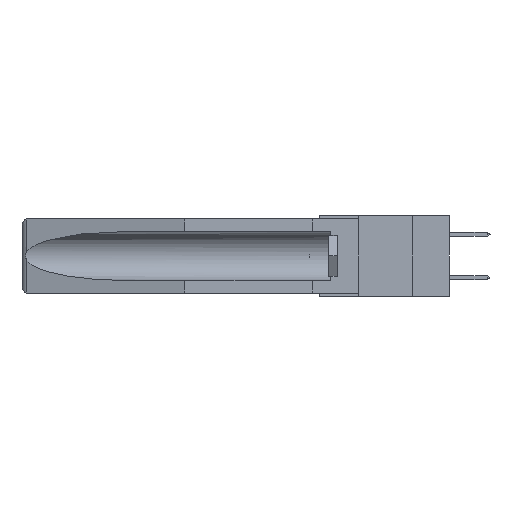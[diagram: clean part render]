
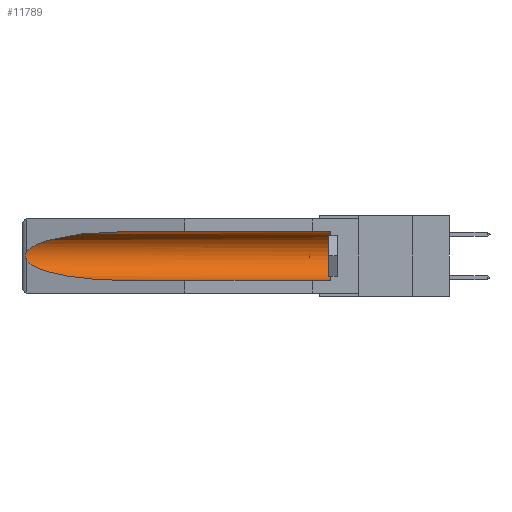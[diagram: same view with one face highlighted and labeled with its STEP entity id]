
A CAD part, left-side view. The second image highlights one B-rep face of the part: STEP entity #11789.
In plain terms, the highlighted cylindrical face has radius 2.857 mm (diameter 5.715 mm), a partial arc.
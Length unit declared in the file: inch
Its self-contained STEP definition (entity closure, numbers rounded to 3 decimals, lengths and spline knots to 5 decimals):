
#1713 = CIRCLE ( 'NONE', #26644, 0.1125 ) ;
#2070 = CARTESIAN_POINT ( 'NONE',  ( 0.26537, 1.52718, -0.14972 ) ) ;
#2084 = LINE ( 'NONE', #13406, #31591 ) ;
#4578 = EDGE_CURVE ( 'NONE', #18161, #4967, #15118, .T. ) ;
#4729 = DIRECTION ( 'NONE',  ( 0., 0., 1. ) ) ;
#4914 = VECTOR ( 'NONE', #30350, 39.37008 ) ;
#4967 = VERTEX_POINT ( 'NONE', #12505 ) ;
#5383 = CARTESIAN_POINT ( 'NONE',  ( 0.26537, 1.52718, -0.19328 ) ) ;
#6079 = EDGE_LOOP ( 'NONE', ( #31868, #26037, #12782, #11870, #13099, #24404 ) ) ;
#6200 = CARTESIAN_POINT ( 'NONE',  ( 0.155, 1.07973, -0.059 ) ) ;
#7453 = CARTESIAN_POINT ( 'NONE',  ( 0.26597, 1.52961, -0.15275 ) ) ;
#8318 = CARTESIAN_POINT ( 'NONE',  ( 0.155, -0.30754, -0.1715 ) ) ;
#9448 = FACE_OUTER_BOUND ( 'NONE', #6079, .T. ) ;
#9853 = CARTESIAN_POINT ( 'NONE',  ( 0.155, 0.126, -0.1715 ) ) ;
#10116 = CARTESIAN_POINT ( 'NONE',  ( 0.2673, 1.5327, -0.16383 ) ) ;
#10233 = CARTESIAN_POINT ( 'NONE',  ( 0.2675, 1.53308, -0.17534 ) ) ;
#10863 = VERTEX_POINT ( 'NONE', #6200 ) ;
#11113 = VERTEX_POINT ( 'NONE', #22282 ) ;
#11429 = CARTESIAN_POINT ( 'NONE',  ( 0.25451, 1.48313, -0.09465 ) ) ;
#11536 = VERTEX_POINT ( 'NONE', #2070 ) ;
#11667 = CARTESIAN_POINT ( 'NONE',  ( 0.26537, 1.52718, -0.14972 ) ) ;
#11789 = ADVANCED_FACE ( 'NONE', ( #9448 ), #16881, .F. ) ;
#11870 = ORIENTED_EDGE ( 'NONE', *, *, #25027, .F. ) ;
#12505 = CARTESIAN_POINT ( 'NONE',  ( 0.155, 1.07973, -0.284 ) ) ;
#12756 = CARTESIAN_POINT ( 'NONE',  ( 0.21114, 1.30732, -0.284 ) ) ;
#12782 = ORIENTED_EDGE ( 'NONE', *, *, #4578, .T. ) ;
#13099 = ORIENTED_EDGE ( 'NONE', *, *, #20640, .T. ) ;
#13406 = CARTESIAN_POINT ( 'NONE',  ( 0.155, -0.30754, -0.059 ) ) ;
#13430 = CARTESIAN_POINT ( 'NONE',  ( 0.26655, 1.53094, -0.18657 ) ) ;
#13573 = CARTESIAN_POINT ( 'NONE',  ( 0.155, 0.126, -0.284 ) ) ;
#13585 = DIRECTION ( 'NONE',  ( 0., 0., 1. ) ) ;
#14086 = DIRECTION ( 'NONE',  ( 0., 1., 0. ) ) ;
#15118 =( BOUNDED_CURVE ( )  B_SPLINE_CURVE ( 3, ( #31991, #29123, #12756, #15468 ),
 .UNSPECIFIED., .F., .F. ) 
 B_SPLINE_CURVE_WITH_KNOTS ( ( 4, 4 ),
 ( 0.1948, 1.5708 ),
 .UNSPECIFIED. ) 
 CURVE ( )  GEOMETRIC_REPRESENTATION_ITEM ( )  RATIONAL_B_SPLINE_CURVE ( ( 1., 0.848, 0.848, 1. ) ) 
 REPRESENTATION_ITEM ( '' )  );
#15468 = CARTESIAN_POINT ( 'NONE',  ( 0.155, 1.07973, -0.284 ) ) ;
#16711 = LINE ( 'NONE', #33012, #4914 ) ;
#16881 = CYLINDRICAL_SURFACE ( 'NONE', #19779, 0.1125 ) ;
#18161 = VERTEX_POINT ( 'NONE', #5383 ) ;
#18174 = VERTEX_POINT ( 'NONE', #13573 ) ;
#18507 = DIRECTION ( 'NONE',  ( 0., -1., 0. ) ) ;
#18749 = EDGE_CURVE ( 'NONE', #10863, #11536, #29467, .T. ) ;
#19779 = AXIS2_PLACEMENT_3D ( 'NONE', #8318, #33048, #13585 ) ;
#19990 = B_SPLINE_CURVE_WITH_KNOTS ( 'NONE', 3,
 ( #21460, #7453, #26871, #10116, #27243, #10233, #26996, #13430, #32783, #24248 ),
 .UNSPECIFIED., .F., .F.,
 ( 4, 2, 2, 2, 4 ),
 ( 0., 0.00029, 0.00058, 0.00087, 0.00117 ),
 .UNSPECIFIED. ) ;
#20640 = EDGE_CURVE ( 'NONE', #18174, #11113, #1713, .T. ) ;
#21197 = CARTESIAN_POINT ( 'NONE',  ( 0.21114, 1.30732, -0.059 ) ) ;
#21460 = CARTESIAN_POINT ( 'NONE',  ( 0.26537, 1.52718, -0.14972 ) ) ;
#22282 = CARTESIAN_POINT ( 'NONE',  ( 0.155, 0.126, -0.059 ) ) ;
#24248 = CARTESIAN_POINT ( 'NONE',  ( 0.26537, 1.52718, -0.19328 ) ) ;
#24404 = ORIENTED_EDGE ( 'NONE', *, *, #32668, .T. ) ;
#25027 = EDGE_CURVE ( 'NONE', #18174, #4967, #16711, .T. ) ;
#26037 = ORIENTED_EDGE ( 'NONE', *, *, #30754, .T. ) ;
#26644 = AXIS2_PLACEMENT_3D ( 'NONE', #9853, #18507, #4729 ) ;
#26871 = CARTESIAN_POINT ( 'NONE',  ( 0.26654, 1.53092, -0.15636 ) ) ;
#26996 = CARTESIAN_POINT ( 'NONE',  ( 0.2673, 1.53269, -0.17917 ) ) ;
#27243 = CARTESIAN_POINT ( 'NONE',  ( 0.2675, 1.53308, -0.16763 ) ) ;
#29123 = CARTESIAN_POINT ( 'NONE',  ( 0.25451, 1.48313, -0.24835 ) ) ;
#29467 =( BOUNDED_CURVE ( )  B_SPLINE_CURVE ( 3, ( #35687, #21197, #11429, #11667 ),
 .UNSPECIFIED., .F., .F. ) 
 B_SPLINE_CURVE_WITH_KNOTS ( ( 4, 4 ),
 ( 4.71239, 6.08839 ),
 .UNSPECIFIED. ) 
 CURVE ( )  GEOMETRIC_REPRESENTATION_ITEM ( )  RATIONAL_B_SPLINE_CURVE ( ( 1., 0.848, 0.848, 1. ) ) 
 REPRESENTATION_ITEM ( '' )  );
#30350 = DIRECTION ( 'NONE',  ( 0., 1., 0. ) ) ;
#30754 = EDGE_CURVE ( 'NONE', #11536, #18161, #19990, .T. ) ;
#31591 = VECTOR ( 'NONE', #14086, 39.37008 ) ;
#31868 = ORIENTED_EDGE ( 'NONE', *, *, #18749, .T. ) ;
#31991 = CARTESIAN_POINT ( 'NONE',  ( 0.26537, 1.52718, -0.19328 ) ) ;
#32668 = EDGE_CURVE ( 'NONE', #11113, #10863, #2084, .T. ) ;
#32783 = CARTESIAN_POINT ( 'NONE',  ( 0.26597, 1.5296, -0.19026 ) ) ;
#33012 = CARTESIAN_POINT ( 'NONE',  ( 0.155, -0.30754, -0.284 ) ) ;
#33048 = DIRECTION ( 'NONE',  ( 0., 1., 0. ) ) ;
#35687 = CARTESIAN_POINT ( 'NONE',  ( 0.155, 1.07973, -0.059 ) ) ;
